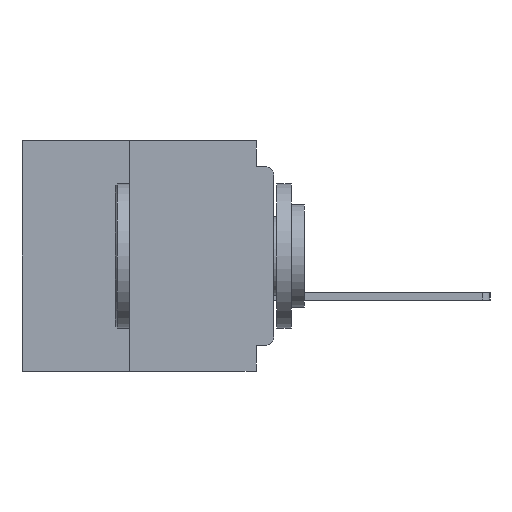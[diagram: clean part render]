
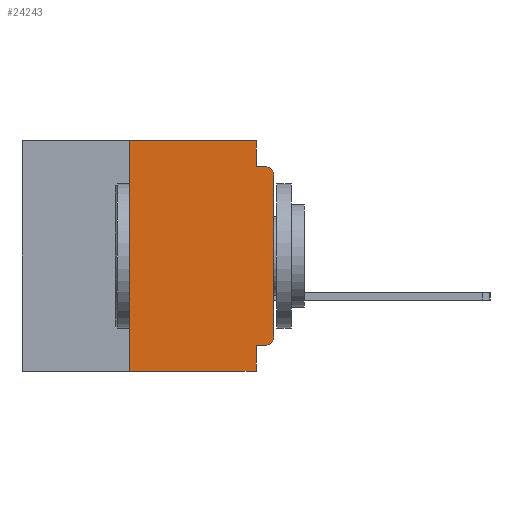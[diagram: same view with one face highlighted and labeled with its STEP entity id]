
A CAD part, left-side view. The second image highlights one B-rep face of the part: STEP entity #24243.
In plain terms, the highlighted planar face has unit normal (-1, 0, 0).
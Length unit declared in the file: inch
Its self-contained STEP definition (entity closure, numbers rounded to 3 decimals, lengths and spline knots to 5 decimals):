
#65 = ORIENTED_EDGE ( 'NONE', *, *, #59692, .F. ) ;
#1595 = VECTOR ( 'NONE', #26162, 39.37008 ) ;
#1801 = VERTEX_POINT ( 'NONE', #39921 ) ;
#2034 = CARTESIAN_POINT ( 'NONE',  ( 0., 0., -0.34 ) ) ;
#3281 = CARTESIAN_POINT ( 'NONE',  ( 0., 0.015, -0.06 ) ) ;
#3620 = FACE_OUTER_BOUND ( 'NONE', #42347, .T. ) ;
#5091 = CARTESIAN_POINT ( 'NONE',  ( 0., 0.031, 0. ) ) ;
#7528 = VECTOR ( 'NONE', #18313, 39.37008 ) ;
#7976 = DIRECTION ( 'NONE',  ( 0., 0., -1. ) ) ;
#8855 = DIRECTION ( 'NONE',  ( 0., 0., -1. ) ) ;
#8982 = CARTESIAN_POINT ( 'NONE',  ( 0., 0.437, 0. ) ) ;
#9972 = VECTOR ( 'NONE', #19657, 39.37008 ) ;
#10094 = VERTEX_POINT ( 'NONE', #37652 ) ;
#10333 = VERTEX_POINT ( 'NONE', #20572 ) ;
#10497 = LINE ( 'NONE', #51269, #7528 ) ;
#10511 = AXIS2_PLACEMENT_3D ( 'NONE', #3281, #36134, #7976 ) ;
#11331 = ORIENTED_EDGE ( 'NONE', *, *, #25181, .F. ) ;
#12431 = ORIENTED_EDGE ( 'NONE', *, *, #24021, .F. ) ;
#14097 = LINE ( 'NONE', #54371, #1595 ) ;
#14417 = EDGE_CURVE ( 'NONE', #54075, #29783, #55129, .T. ) ;
#14939 = CARTESIAN_POINT ( 'NONE',  ( 0., 0.031, -0.4 ) ) ;
#15030 = CARTESIAN_POINT ( 'NONE',  ( 0., 0.015, -0.355 ) ) ;
#15469 = VERTEX_POINT ( 'NONE', #15030 ) ;
#18313 = DIRECTION ( 'NONE',  ( 0., 0., 1. ) ) ;
#18918 = CARTESIAN_POINT ( 'NONE',  ( 0., 0.25, -0.4 ) ) ;
#19490 = CARTESIAN_POINT ( 'NONE',  ( 0., 0.015, -0.34 ) ) ;
#19657 = DIRECTION ( 'NONE',  ( 0., 0., -1. ) ) ;
#20129 = LINE ( 'NONE', #8982, #31165 ) ;
#20504 = ORIENTED_EDGE ( 'NONE', *, *, #56204, .T. ) ;
#20572 = CARTESIAN_POINT ( 'NONE',  ( 0., 0.015, -0.045 ) ) ;
#21609 = VECTOR ( 'NONE', #41658, 39.37008 ) ;
#22144 = CARTESIAN_POINT ( 'NONE',  ( 0., 0.031, -0.4 ) ) ;
#22859 = CARTESIAN_POINT ( 'NONE',  ( 0., 0.031, 0. ) ) ;
#23759 = PLANE ( 'NONE',  #36243 ) ;
#24021 = EDGE_CURVE ( 'NONE', #53379, #1801, #40426, .T. ) ;
#24072 = LINE ( 'NONE', #54326, #25567 ) ;
#24158 = CIRCLE ( 'NONE', #10511, 0.015 ) ;
#24214 = DIRECTION ( 'NONE',  ( 0., 0., -1. ) ) ;
#24243 = ADVANCED_FACE ( 'NONE', ( #3620 ), #23759, .F. ) ;
#25181 = EDGE_CURVE ( 'NONE', #29783, #10333, #24072, .T. ) ;
#25567 = VECTOR ( 'NONE', #30858, 39.37008 ) ;
#25571 = EDGE_CURVE ( 'NONE', #15469, #34978, #38006, .T. ) ;
#26162 = DIRECTION ( 'NONE',  ( 0., -1., 0. ) ) ;
#26904 = DIRECTION ( 'NONE',  ( 0., 0., 1. ) ) ;
#27431 = ORIENTED_EDGE ( 'NONE', *, *, #32549, .T. ) ;
#28491 = DIRECTION ( 'NONE',  ( 0., 0., -1. ) ) ;
#29783 = VERTEX_POINT ( 'NONE', #30315 ) ;
#30315 = CARTESIAN_POINT ( 'NONE',  ( 0., 0.031, -0.045 ) ) ;
#30605 = EDGE_CURVE ( 'NONE', #34978, #10094, #10497, .T. ) ;
#30858 = DIRECTION ( 'NONE',  ( 0., -1., 0. ) ) ;
#31165 = VECTOR ( 'NONE', #46633, 39.37008 ) ;
#32549 = EDGE_CURVE ( 'NONE', #53379, #52311, #14097, .T. ) ;
#34978 = VERTEX_POINT ( 'NONE', #2034 ) ;
#35747 = EDGE_CURVE ( 'NONE', #52534, #52311, #60001, .T. ) ;
#36134 = DIRECTION ( 'NONE',  ( -1., 0., 0. ) ) ;
#36243 = AXIS2_PLACEMENT_3D ( 'NONE', #51970, #56664, #28491 ) ;
#36934 = CARTESIAN_POINT ( 'NONE',  ( 0., 0., -0.355 ) ) ;
#37652 = CARTESIAN_POINT ( 'NONE',  ( 0., 0., -0.06 ) ) ;
#38006 = CIRCLE ( 'NONE', #47365, 0.015 ) ;
#38225 = ORIENTED_EDGE ( 'NONE', *, *, #35747, .F. ) ;
#38954 = VECTOR ( 'NONE', #26904, 39.37008 ) ;
#39921 = CARTESIAN_POINT ( 'NONE',  ( 0., 0.25, 0. ) ) ;
#40426 = LINE ( 'NONE', #45603, #38954 ) ;
#41658 = DIRECTION ( 'NONE',  ( 0., 1., 0. ) ) ;
#42347 = EDGE_LOOP ( 'NONE', ( #48423, #20504, #11331, #51140, #46974, #12431, #27431, #38225, #65, #47732 ) ) ;
#42607 = VECTOR ( 'NONE', #8855, 39.37008 ) ;
#45603 = CARTESIAN_POINT ( 'NONE',  ( 0., 0.25, -0.4 ) ) ;
#46633 = DIRECTION ( 'NONE',  ( 0., -1., 0. ) ) ;
#46974 = ORIENTED_EDGE ( 'NONE', *, *, #59716, .F. ) ;
#47365 = AXIS2_PLACEMENT_3D ( 'NONE', #19490, #52431, #24214 ) ;
#47732 = ORIENTED_EDGE ( 'NONE', *, *, #25571, .T. ) ;
#48423 = ORIENTED_EDGE ( 'NONE', *, *, #30605, .T. ) ;
#51140 = ORIENTED_EDGE ( 'NONE', *, *, #14417, .F. ) ;
#51269 = CARTESIAN_POINT ( 'NONE',  ( 0., 0., 0. ) ) ;
#51970 = CARTESIAN_POINT ( 'NONE',  ( 0., 0.437, 0. ) ) ;
#52311 = VERTEX_POINT ( 'NONE', #22144 ) ;
#52431 = DIRECTION ( 'NONE',  ( -1., 0., 0. ) ) ;
#52534 = VERTEX_POINT ( 'NONE', #54208 ) ;
#53379 = VERTEX_POINT ( 'NONE', #18918 ) ;
#54075 = VERTEX_POINT ( 'NONE', #5091 ) ;
#54208 = CARTESIAN_POINT ( 'NONE',  ( 0., 0.031, -0.355 ) ) ;
#54326 = CARTESIAN_POINT ( 'NONE',  ( 0., 0., -0.045 ) ) ;
#54371 = CARTESIAN_POINT ( 'NONE',  ( 0., 0.437, -0.4 ) ) ;
#55129 = LINE ( 'NONE', #22859, #42607 ) ;
#56204 = EDGE_CURVE ( 'NONE', #10094, #10333, #24158, .T. ) ;
#56664 = DIRECTION ( 'NONE',  ( 1., 0., 0. ) ) ;
#59106 = LINE ( 'NONE', #36934, #21609 ) ;
#59692 = EDGE_CURVE ( 'NONE', #15469, #52534, #59106, .T. ) ;
#59716 = EDGE_CURVE ( 'NONE', #1801, #54075, #20129, .T. ) ;
#60001 = LINE ( 'NONE', #14939, #9972 ) ;
